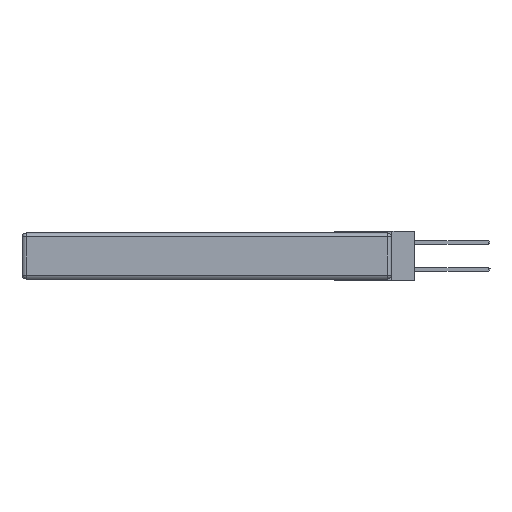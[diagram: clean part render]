
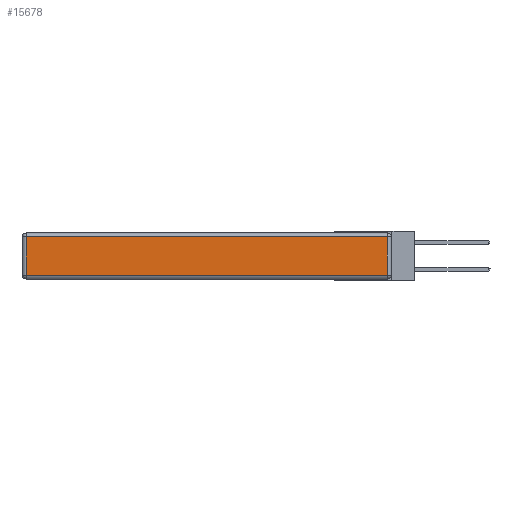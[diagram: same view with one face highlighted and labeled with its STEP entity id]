
A CAD part, left-side view. The second image highlights one B-rep face of the part: STEP entity #15678.
In plain terms, the highlighted planar face has unit normal (-1, 0, 0).
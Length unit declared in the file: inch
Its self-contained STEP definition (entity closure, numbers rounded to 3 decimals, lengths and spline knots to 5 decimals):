
#22 = VERTEX_POINT ( 'NONE', #3128 ) ;
#29 = DIRECTION ( 'NONE',  ( 0., -1., 0. ) ) ;
#1074 = AXIS2_PLACEMENT_3D ( 'NONE', #10645, #20231, #12620 ) ;
#1287 = LINE ( 'NONE', #5980, #19052 ) ;
#3044 = ORIENTED_EDGE ( 'NONE', *, *, #5916, .T. ) ;
#3128 = CARTESIAN_POINT ( 'NONE',  ( 0., 2.72, -0.313 ) ) ;
#3392 = FACE_OUTER_BOUND ( 'NONE', #4132, .T. ) ;
#4132 = EDGE_LOOP ( 'NONE', ( #3044, #11407, #19531, #15363 ) ) ;
#4810 = VECTOR ( 'NONE', #15300, 39.37008 ) ;
#5838 = CARTESIAN_POINT ( 'NONE',  ( 0., 2.72, -0.343 ) ) ;
#5916 = EDGE_CURVE ( 'NONE', #22, #15847, #1287, .T. ) ;
#5980 = CARTESIAN_POINT ( 'NONE',  ( 0., 0., -0.313 ) ) ;
#6651 = CARTESIAN_POINT ( 'NONE',  ( 0., 2.72, -0.03 ) ) ;
#8212 = LINE ( 'NONE', #20452, #21528 ) ;
#9186 = DIRECTION ( 'NONE',  ( 0., 0., 1. ) ) ;
#9207 = CARTESIAN_POINT ( 'NONE',  ( 0., 0.03, -0.313 ) ) ;
#10645 = CARTESIAN_POINT ( 'NONE',  ( 0., 0., -0.343 ) ) ;
#10705 = EDGE_CURVE ( 'NONE', #14580, #22, #20072, .T. ) ;
#11407 = ORIENTED_EDGE ( 'NONE', *, *, #22918, .T. ) ;
#12620 = DIRECTION ( 'NONE',  ( 0., 0., 1. ) ) ;
#13732 = CARTESIAN_POINT ( 'NONE',  ( 0., 2.75, -0.03 ) ) ;
#14421 = CARTESIAN_POINT ( 'NONE',  ( 0., 0.03, -0.03 ) ) ;
#14580 = VERTEX_POINT ( 'NONE', #6651 ) ;
#15275 = DIRECTION ( 'NONE',  ( 0., 0., -1. ) ) ;
#15300 = DIRECTION ( 'NONE',  ( 0., 1., 0. ) ) ;
#15363 = ORIENTED_EDGE ( 'NONE', *, *, #10705, .T. ) ;
#15678 = ADVANCED_FACE ( 'NONE', ( #3392 ), #23697, .T. ) ;
#15847 = VERTEX_POINT ( 'NONE', #9207 ) ;
#16801 = VECTOR ( 'NONE', #15275, 39.37008 ) ;
#17585 = VERTEX_POINT ( 'NONE', #14421 ) ;
#18832 = EDGE_CURVE ( 'NONE', #17585, #14580, #22007, .T. ) ;
#19052 = VECTOR ( 'NONE', #29, 39.37008 ) ;
#19531 = ORIENTED_EDGE ( 'NONE', *, *, #18832, .T. ) ;
#20072 = LINE ( 'NONE', #5838, #16801 ) ;
#20231 = DIRECTION ( 'NONE',  ( -1., 0., 0. ) ) ;
#20452 = CARTESIAN_POINT ( 'NONE',  ( 0., 0.03, -0.343 ) ) ;
#21528 = VECTOR ( 'NONE', #9186, 39.37008 ) ;
#22007 = LINE ( 'NONE', #13732, #4810 ) ;
#22918 = EDGE_CURVE ( 'NONE', #15847, #17585, #8212, .T. ) ;
#23697 = PLANE ( 'NONE',  #1074 ) ;
